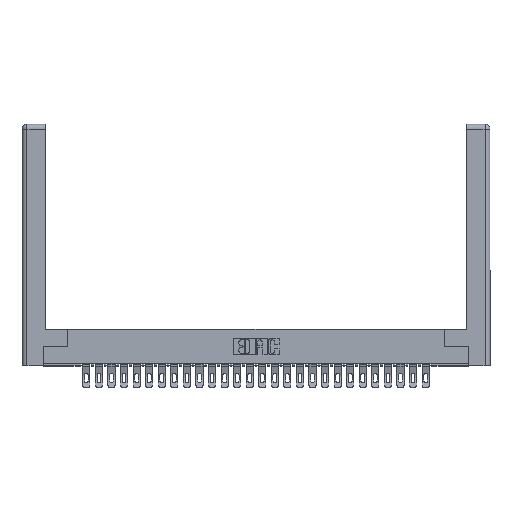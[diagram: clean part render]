
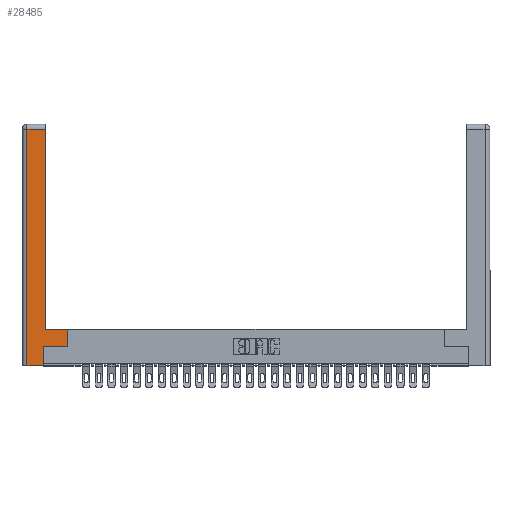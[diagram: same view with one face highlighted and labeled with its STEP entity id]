
A CAD part, top view. The second image highlights one B-rep face of the part: STEP entity #28485.
In plain terms, the highlighted planar face has unit normal (0, 0, 1).
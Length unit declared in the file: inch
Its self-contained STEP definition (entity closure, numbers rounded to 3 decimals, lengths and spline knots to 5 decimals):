
#312 = DIRECTION ( 'NONE',  ( 0., 1., 0. ) ) ;
#695 = EDGE_CURVE ( 'NONE', #21424, #25671, #23169, .T. ) ;
#924 = CARTESIAN_POINT ( 'NONE',  ( 0.0615, 2.94, 0. ) ) ;
#1403 = VECTOR ( 'NONE', #312, 39.37008 ) ;
#2012 = EDGE_CURVE ( 'NONE', #7921, #14988, #8997, .T. ) ;
#2556 = ORIENTED_EDGE ( 'NONE', *, *, #24048, .T. ) ;
#2928 = CARTESIAN_POINT ( 'NONE',  ( 0.295, 0.45, 0. ) ) ;
#3201 = PLANE ( 'NONE',  #31418 ) ;
#3508 = EDGE_CURVE ( 'NONE', #28057, #7921, #8385, .T. ) ;
#4473 = CARTESIAN_POINT ( 'NONE',  ( 0.0615, 2.94, 0. ) ) ;
#5323 = DIRECTION ( 'NONE',  ( 0., 1., 0. ) ) ;
#5625 = VECTOR ( 'NONE', #5323, 39.37008 ) ;
#5727 = CARTESIAN_POINT ( 'NONE',  ( 0.565, 0.45, 0. ) ) ;
#5802 = DIRECTION ( 'NONE',  ( 0., 0., -1. ) ) ;
#6285 = DIRECTION ( 'NONE',  ( 0., -1., 0. ) ) ;
#6764 = VECTOR ( 'NONE', #17727, 39.37008 ) ;
#7865 = CARTESIAN_POINT ( 'NONE',  ( 0.265, 0.245, 0. ) ) ;
#7921 = VERTEX_POINT ( 'NONE', #4473 ) ;
#8385 = LINE ( 'NONE', #924, #20768 ) ;
#8644 = LINE ( 'NONE', #8757, #1403 ) ;
#8757 = CARTESIAN_POINT ( 'NONE',  ( 0.295, 3., 0. ) ) ;
#8997 = LINE ( 'NONE', #15002, #31585 ) ;
#9095 = CARTESIAN_POINT ( 'NONE',  ( 0.565, 0.45, 0. ) ) ;
#10013 = ORIENTED_EDGE ( 'NONE', *, *, #18956, .T. ) ;
#10826 = DIRECTION ( 'NONE',  ( -1., 0., 0. ) ) ;
#12050 = VECTOR ( 'NONE', #25293, 39.37008 ) ;
#12255 = CARTESIAN_POINT ( 'NONE',  ( 0.295, 0.45, 0. ) ) ;
#12873 = EDGE_CURVE ( 'NONE', #19459, #28057, #8644, .T. ) ;
#13150 = CARTESIAN_POINT ( 'NONE',  ( 0.0615, 0., 0. ) ) ;
#13308 = LINE ( 'NONE', #2928, #28628 ) ;
#14003 = CARTESIAN_POINT ( 'NONE',  ( 0.265, 0.245, 0. ) ) ;
#14041 = DIRECTION ( 'NONE',  ( -1., 0., 0. ) ) ;
#14988 = VERTEX_POINT ( 'NONE', #13150 ) ;
#14993 = CARTESIAN_POINT ( 'NONE',  ( 0.265, 0., 0. ) ) ;
#15002 = CARTESIAN_POINT ( 'NONE',  ( 0.0615, 0., 0. ) ) ;
#16589 = EDGE_LOOP ( 'NONE', ( #31611, #16850, #31336, #34352, #10013, #16711, #26711, #2556 ) ) ;
#16711 = ORIENTED_EDGE ( 'NONE', *, *, #695, .T. ) ;
#16850 = ORIENTED_EDGE ( 'NONE', *, *, #3508, .T. ) ;
#16871 = CARTESIAN_POINT ( 'NONE',  ( 0.565, 0.245, 0. ) ) ;
#17611 = DIRECTION ( 'NONE',  ( -1., 0., 0. ) ) ;
#17727 = DIRECTION ( 'NONE',  ( 1., 0., 0. ) ) ;
#17773 = CARTESIAN_POINT ( 'NONE',  ( 0.295, 2.94, 0. ) ) ;
#18956 = EDGE_CURVE ( 'NONE', #33115, #21424, #26973, .T. ) ;
#19342 = VECTOR ( 'NONE', #28263, 39.37008 ) ;
#19459 = VERTEX_POINT ( 'NONE', #12255 ) ;
#20768 = VECTOR ( 'NONE', #17611, 39.37008 ) ;
#20939 = EDGE_CURVE ( 'NONE', #14988, #33115, #26387, .T. ) ;
#21424 = VERTEX_POINT ( 'NONE', #14003 ) ;
#21974 = FACE_OUTER_BOUND ( 'NONE', #16589, .T. ) ;
#22826 = CARTESIAN_POINT ( 'NONE',  ( 0.565, 0.245, 0. ) ) ;
#23169 = LINE ( 'NONE', #22826, #19342 ) ;
#24048 = EDGE_CURVE ( 'NONE', #29047, #19459, #13308, .T. ) ;
#24826 = LINE ( 'NONE', #9095, #12050 ) ;
#25293 = DIRECTION ( 'NONE',  ( 0., 1., 0. ) ) ;
#25671 = VERTEX_POINT ( 'NONE', #16871 ) ;
#26387 = LINE ( 'NONE', #14993, #6764 ) ;
#26711 = ORIENTED_EDGE ( 'NONE', *, *, #30417, .T. ) ;
#26827 = CARTESIAN_POINT ( 'NONE',  ( 0.265, 0., 0. ) ) ;
#26973 = LINE ( 'NONE', #7865, #5625 ) ;
#28057 = VERTEX_POINT ( 'NONE', #17773 ) ;
#28263 = DIRECTION ( 'NONE',  ( 1., 0., 0. ) ) ;
#28485 = ADVANCED_FACE ( 'NONE', ( #21974 ), #3201, .F. ) ;
#28628 = VECTOR ( 'NONE', #10826, 39.37008 ) ;
#29047 = VERTEX_POINT ( 'NONE', #5727 ) ;
#30334 = CARTESIAN_POINT ( 'NONE',  ( 0., 0., 0. ) ) ;
#30417 = EDGE_CURVE ( 'NONE', #25671, #29047, #24826, .T. ) ;
#31336 = ORIENTED_EDGE ( 'NONE', *, *, #2012, .T. ) ;
#31418 = AXIS2_PLACEMENT_3D ( 'NONE', #30334, #5802, #14041 ) ;
#31585 = VECTOR ( 'NONE', #6285, 39.37008 ) ;
#31611 = ORIENTED_EDGE ( 'NONE', *, *, #12873, .T. ) ;
#33115 = VERTEX_POINT ( 'NONE', #26827 ) ;
#34352 = ORIENTED_EDGE ( 'NONE', *, *, #20939, .T. ) ;
